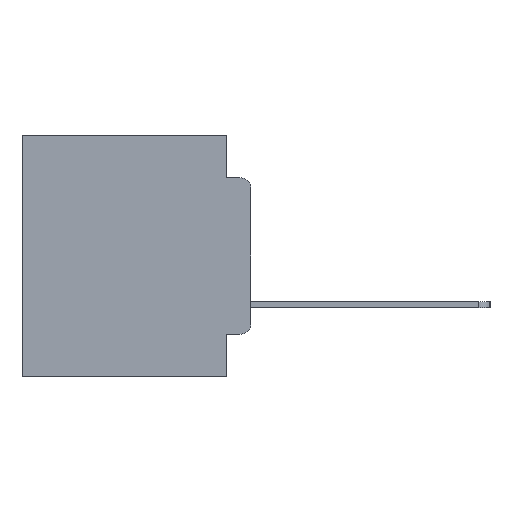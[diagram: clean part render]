
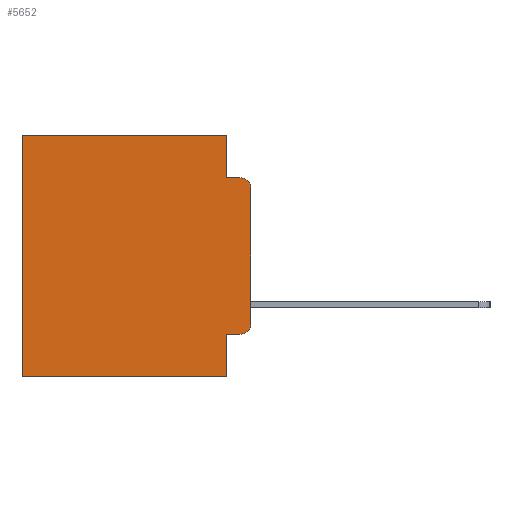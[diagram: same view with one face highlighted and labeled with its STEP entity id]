
A CAD part, left-side view. The second image highlights one B-rep face of the part: STEP entity #5652.
In plain terms, the highlighted planar face has unit normal (-1, 0, 0).
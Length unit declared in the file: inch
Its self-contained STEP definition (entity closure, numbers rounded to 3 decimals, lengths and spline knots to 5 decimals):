
#1130 = CARTESIAN_POINT ( 'NONE',  ( 0.298, 0.051, -0.4115 ) ) ;
#1275 = FACE_OUTER_BOUND ( 'NONE', #12603, .T. ) ;
#1306 = VECTOR ( 'NONE', #17040, 39.37008 ) ;
#1791 = CARTESIAN_POINT ( 'NONE',  ( 0.298, 0., 0. ) ) ;
#1883 = CARTESIAN_POINT ( 'NONE',  ( 0.298, 0.051, 0. ) ) ;
#2068 = CARTESIAN_POINT ( 'NONE',  ( 0.298, 0.473, 0. ) ) ;
#2194 = CARTESIAN_POINT ( 'NONE',  ( 0.298, 0.473, 0. ) ) ;
#2870 = CARTESIAN_POINT ( 'NONE',  ( 0.298, 0.051, -0.0885 ) ) ;
#2907 = CARTESIAN_POINT ( 'NONE',  ( 0.298, 0.051, -0.0885 ) ) ;
#3474 = DIRECTION ( 'NONE',  ( -1., 0., 0. ) ) ;
#3702 = DIRECTION ( 'NONE',  ( 0., -1., 0. ) ) ;
#3975 = ORIENTED_EDGE ( 'NONE', *, *, #21970, .F. ) ;
#4234 = CARTESIAN_POINT ( 'NONE',  ( 0.298, 0.051, -0.5 ) ) ;
#4390 = DIRECTION ( 'NONE',  ( 0., 1., 0. ) ) ;
#4407 = CARTESIAN_POINT ( 'NONE',  ( 0.298, 0.051, -0.4115 ) ) ;
#4627 = VERTEX_POINT ( 'NONE', #2068 ) ;
#5343 = VECTOR ( 'NONE', #16438, 39.37008 ) ;
#5652 = ADVANCED_FACE ( 'NONE', ( #1275 ), #22883, .F. ) ;
#5773 = ORIENTED_EDGE ( 'NONE', *, *, #14325, .F. ) ;
#5806 = CARTESIAN_POINT ( 'NONE',  ( 0.298, 0.051, 0. ) ) ;
#6309 = VECTOR ( 'NONE', #4390, 39.37008 ) ;
#7985 = ORIENTED_EDGE ( 'NONE', *, *, #13289, .F. ) ;
#8519 = ORIENTED_EDGE ( 'NONE', *, *, #13370, .F. ) ;
#8654 = CARTESIAN_POINT ( 'NONE',  ( 0.298, 0.02, -0.4115 ) ) ;
#8868 = VERTEX_POINT ( 'NONE', #26204 ) ;
#9553 = LINE ( 'NONE', #2194, #21750 ) ;
#9634 = EDGE_CURVE ( 'NONE', #15919, #4627, #25206, .T. ) ;
#9936 = VECTOR ( 'NONE', #3702, 39.37008 ) ;
#10635 = VECTOR ( 'NONE', #12814, 39.37008 ) ;
#11392 = ORIENTED_EDGE ( 'NONE', *, *, #9634, .T. ) ;
#11694 = VECTOR ( 'NONE', #24172, 39.37008 ) ;
#11957 = CARTESIAN_POINT ( 'NONE',  ( 0.298, 0., -0.3915 ) ) ;
#12165 = LINE ( 'NONE', #2870, #10635 ) ;
#12185 = DIRECTION ( 'NONE',  ( 0., 0., -1. ) ) ;
#12603 = EDGE_LOOP ( 'NONE', ( #5773, #25692, #8519, #7985, #11392, #22111, #3975, #26105, #22487, #17491 ) ) ;
#12764 = VERTEX_POINT ( 'NONE', #4407 ) ;
#12814 = DIRECTION ( 'NONE',  ( 0., -1., 0. ) ) ;
#12815 = CARTESIAN_POINT ( 'NONE',  ( 0.298, 0., -0.5 ) ) ;
#12956 = EDGE_CURVE ( 'NONE', #13525, #13213, #13676, .T. ) ;
#12982 = CARTESIAN_POINT ( 'NONE',  ( 0.298, 0., 0. ) ) ;
#13001 = EDGE_CURVE ( 'NONE', #12764, #13525, #16908, .T. ) ;
#13155 = EDGE_CURVE ( 'NONE', #12764, #19119, #18651, .T. ) ;
#13213 = VERTEX_POINT ( 'NONE', #11957 ) ;
#13239 = EDGE_CURVE ( 'NONE', #4627, #13648, #9553, .T. ) ;
#13289 = EDGE_CURVE ( 'NONE', #15919, #25694, #19706, .T. ) ;
#13370 = EDGE_CURVE ( 'NONE', #25694, #19936, #12165, .T. ) ;
#13525 = VERTEX_POINT ( 'NONE', #8654 ) ;
#13648 = VERTEX_POINT ( 'NONE', #13901 ) ;
#13676 = CIRCLE ( 'NONE', #28927, 0.02 ) ;
#13901 = CARTESIAN_POINT ( 'NONE',  ( 0.298, 0.473, -0.5 ) ) ;
#14094 = EDGE_CURVE ( 'NONE', #8868, #19936, #25997, .T. ) ;
#14305 = CARTESIAN_POINT ( 'NONE',  ( 0.298, 0.02, -0.1085 ) ) ;
#14325 = EDGE_CURVE ( 'NONE', #8868, #13213, #17877, .T. ) ;
#15919 = VERTEX_POINT ( 'NONE', #5806 ) ;
#16403 = DIRECTION ( 'NONE',  ( 0., 0., -1. ) ) ;
#16438 = DIRECTION ( 'NONE',  ( 0., 0., -1. ) ) ;
#16463 = DIRECTION ( 'NONE',  ( 1., 0., 0. ) ) ;
#16607 = DIRECTION ( 'NONE',  ( 0., 0., -1. ) ) ;
#16908 = LINE ( 'NONE', #1130, #9936 ) ;
#17040 = DIRECTION ( 'NONE',  ( 0., 0., -1. ) ) ;
#17438 = VECTOR ( 'NONE', #26132, 39.37008 ) ;
#17491 = ORIENTED_EDGE ( 'NONE', *, *, #12956, .T. ) ;
#17842 = AXIS2_PLACEMENT_3D ( 'NONE', #24384, #16463, #16403 ) ;
#17859 = CARTESIAN_POINT ( 'NONE',  ( 0.298, 0.02, -0.3915 ) ) ;
#17877 = LINE ( 'NONE', #12982, #11694 ) ;
#18651 = LINE ( 'NONE', #1883, #5343 ) ;
#19119 = VERTEX_POINT ( 'NONE', #4234 ) ;
#19706 = LINE ( 'NONE', #21524, #1306 ) ;
#19936 = VERTEX_POINT ( 'NONE', #27558 ) ;
#20114 = DIRECTION ( 'NONE',  ( 0., 0., -1. ) ) ;
#21524 = CARTESIAN_POINT ( 'NONE',  ( 0.298, 0.051, 0. ) ) ;
#21750 = VECTOR ( 'NONE', #12185, 39.37008 ) ;
#21970 = EDGE_CURVE ( 'NONE', #19119, #13648, #23273, .T. ) ;
#22111 = ORIENTED_EDGE ( 'NONE', *, *, #13239, .T. ) ;
#22487 = ORIENTED_EDGE ( 'NONE', *, *, #13001, .T. ) ;
#22883 = PLANE ( 'NONE',  #17842 ) ;
#23273 = LINE ( 'NONE', #12815, #17438 ) ;
#24172 = DIRECTION ( 'NONE',  ( 0., 0., -1. ) ) ;
#24384 = CARTESIAN_POINT ( 'NONE',  ( 0.298, 0., 0. ) ) ;
#25206 = LINE ( 'NONE', #1791, #6309 ) ;
#25692 = ORIENTED_EDGE ( 'NONE', *, *, #14094, .T. ) ;
#25694 = VERTEX_POINT ( 'NONE', #2907 ) ;
#25997 = CIRCLE ( 'NONE', #28618, 0.02 ) ;
#26105 = ORIENTED_EDGE ( 'NONE', *, *, #13155, .F. ) ;
#26132 = DIRECTION ( 'NONE',  ( 0., 1., 0. ) ) ;
#26204 = CARTESIAN_POINT ( 'NONE',  ( 0.298, 0., -0.1085 ) ) ;
#27558 = CARTESIAN_POINT ( 'NONE',  ( 0.298, 0.02, -0.0885 ) ) ;
#28618 = AXIS2_PLACEMENT_3D ( 'NONE', #14305, #29407, #16607 ) ;
#28927 = AXIS2_PLACEMENT_3D ( 'NONE', #17859, #3474, #20114 ) ;
#29407 = DIRECTION ( 'NONE',  ( -1., 0., 0. ) ) ;
